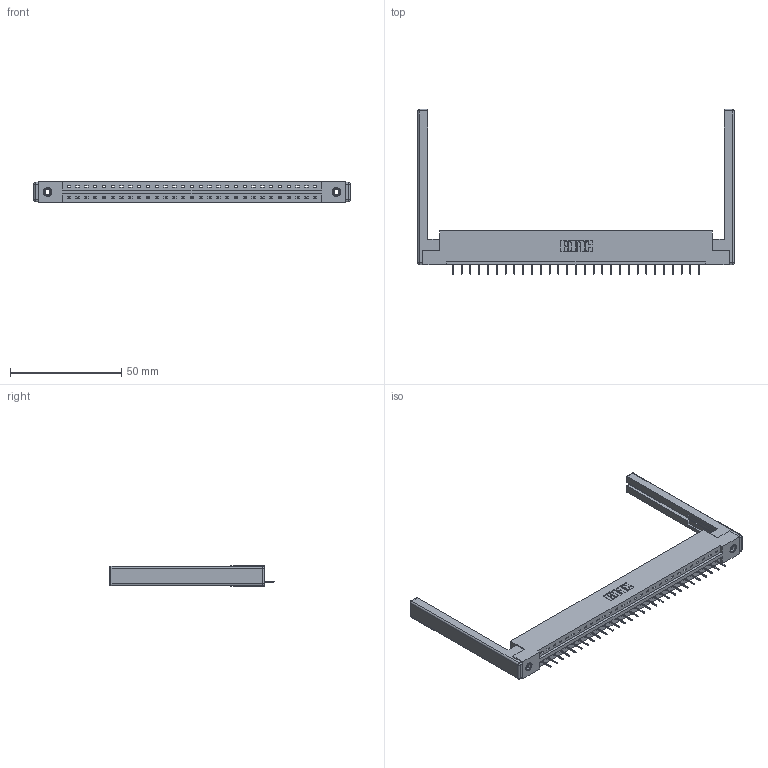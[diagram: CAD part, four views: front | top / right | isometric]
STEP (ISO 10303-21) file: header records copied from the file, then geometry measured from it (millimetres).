
FILE_DESCRIPTION (( 'STEP AP203' ), '1' );
FILE_NAME ('337-029-524-168.STEP', '2019-09-30T22:15:41', ( '' ), ( '' ), 'SwSTEP 2.0', 'SolidWorks 2016', '' );
FILE_SCHEMA (( 'CONFIG_CONTROL_DESIGN' ));
Length unit declared in the file: inch
Products named in the file (5): 345-250-001_345-250-001-102; 337-029-524-168; 337 Part_Flush Mounting Lugs - 0.156 Dia-TI; 345-292-001_345-293-124; 307-220-068
Assembly tree (34 placements, depth 2):
  337-029-524-168
    337 Part_Flush Mounting Lugs - 0.156 Dia-TI
    345-292-001_345-293-124  x29
    345-250-001_345-250-001-102  x2
    307-220-068  x2
Bounding box: 142.34 x 74.43 x 9.4 mm (x, y, z)
Volume: 18908 mm3; surface area: 18618.6 mm2
Topology: 34 solids, 34 shells, 2182 faces, 6269 edges, 4042 vertices
Faces by surface type: plane 1666, cylinder 492, cone 12, sphere 8, torus 4
Entity records: 26072 total; most frequent: CARTESIAN_POINT 4494, ORIENTED_EDGE 4448, DIRECTION 3884, EDGE_CURVE 2224, LINE 2050, VECTOR 2050, VERTEX_POINT 1470, AXIS2_PLACEMENT_3D 917
